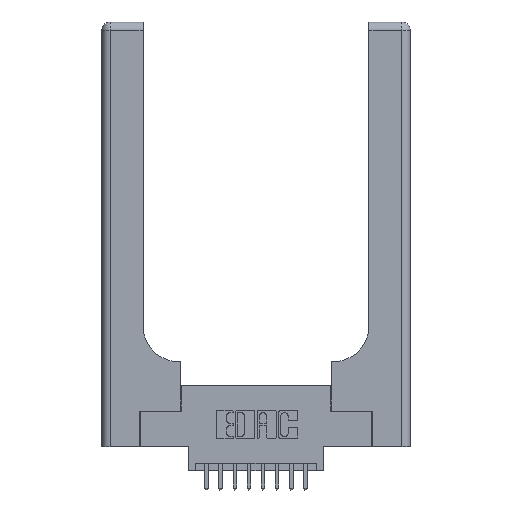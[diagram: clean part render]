
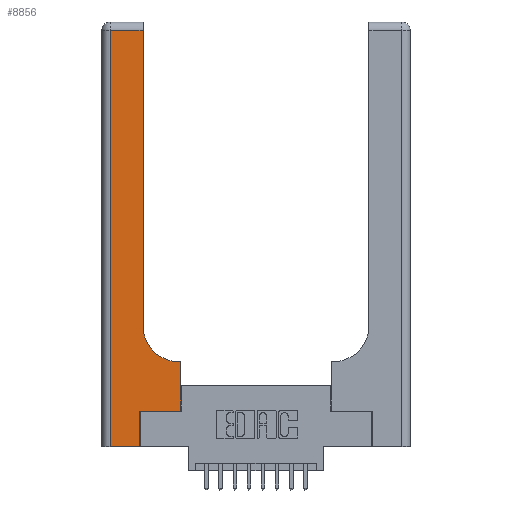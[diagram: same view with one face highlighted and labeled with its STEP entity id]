
A CAD part, top view. The second image highlights one B-rep face of the part: STEP entity #8856.
In plain terms, the highlighted planar face has unit normal (0, 0, 1).
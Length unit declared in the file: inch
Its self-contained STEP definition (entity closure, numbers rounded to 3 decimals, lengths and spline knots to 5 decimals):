
#117 = DIRECTION ( 'NONE',  ( 0., -1., 0. ) ) ;
#145 = CARTESIAN_POINT ( 'NONE',  ( 0.2915, 3., 0.37 ) ) ;
#798 = DIRECTION ( 'NONE',  ( -1., 0., 0. ) ) ;
#891 = VERTEX_POINT ( 'NONE', #4450 ) ;
#1082 = ORIENTED_EDGE ( 'NONE', *, *, #5301, .T. ) ;
#1162 = PLANE ( 'NONE',  #9808 ) ;
#1988 = LINE ( 'NONE', #13821, #11573 ) ;
#2045 = VECTOR ( 'NONE', #13117, 39.37008 ) ;
#2128 = DIRECTION ( 'NONE',  ( 1., 0., 0. ) ) ;
#2146 = DIRECTION ( 'NONE',  ( 0., 0., -1. ) ) ;
#2162 = CARTESIAN_POINT ( 'NONE',  ( 0.5415, 0.85, 0.37 ) ) ;
#2391 = VERTEX_POINT ( 'NONE', #8652 ) ;
#2441 = ORIENTED_EDGE ( 'NONE', *, *, #9948, .T. ) ;
#2488 = VECTOR ( 'NONE', #12244, 39.37008 ) ;
#2704 = DIRECTION ( 'NONE',  ( 0., 1., 0. ) ) ;
#2963 = CARTESIAN_POINT ( 'NONE',  ( 0.06, 2.94, 0.37 ) ) ;
#2995 = ORIENTED_EDGE ( 'NONE', *, *, #10984, .T. ) ;
#3245 = EDGE_CURVE ( 'NONE', #11311, #9466, #4702, .T. ) ;
#4249 = CARTESIAN_POINT ( 'NONE',  ( 0.06, 0., 0.37 ) ) ;
#4450 = CARTESIAN_POINT ( 'NONE',  ( 0.269, 0.25, 0.37 ) ) ;
#4457 = CARTESIAN_POINT ( 'NONE',  ( 0., 2.94, 0.37 ) ) ;
#4702 = CIRCLE ( 'NONE', #12982, 0.25 ) ;
#4974 = DIRECTION ( 'NONE',  ( -1., 0., 0. ) ) ;
#5070 = CARTESIAN_POINT ( 'NONE',  ( 0.2915, 0.85, 0.37 ) ) ;
#5249 = CARTESIAN_POINT ( 'NONE',  ( 0.269, 0., 0.37 ) ) ;
#5293 = CARTESIAN_POINT ( 'NONE',  ( 0.5585, 0.25, 0.37 ) ) ;
#5301 = EDGE_CURVE ( 'NONE', #7174, #891, #6236, .T. ) ;
#5472 = ORIENTED_EDGE ( 'NONE', *, *, #3245, .T. ) ;
#5630 = DIRECTION ( 'NONE',  ( 0., 1., 0. ) ) ;
#5690 = CARTESIAN_POINT ( 'NONE',  ( 0., 0., 0.37 ) ) ;
#5772 = LINE ( 'NONE', #145, #11979 ) ;
#5844 = DIRECTION ( 'NONE',  ( 1., 0., 0. ) ) ;
#5846 = CARTESIAN_POINT ( 'NONE',  ( 0.2915, 0.6, 0.37 ) ) ;
#5911 = EDGE_CURVE ( 'NONE', #2391, #11311, #10860, .T. ) ;
#6059 = VERTEX_POINT ( 'NONE', #5293 ) ;
#6215 = VECTOR ( 'NONE', #14359, 39.37008 ) ;
#6236 = LINE ( 'NONE', #8531, #2488 ) ;
#6268 = EDGE_CURVE ( 'NONE', #7899, #6760, #14922, .T. ) ;
#6528 = ORIENTED_EDGE ( 'NONE', *, *, #5911, .T. ) ;
#6760 = VERTEX_POINT ( 'NONE', #2963 ) ;
#7079 = FACE_OUTER_BOUND ( 'NONE', #8393, .T. ) ;
#7174 = VERTEX_POINT ( 'NONE', #5249 ) ;
#7430 = CARTESIAN_POINT ( 'NONE',  ( 0., 3., 0.37 ) ) ;
#7899 = VERTEX_POINT ( 'NONE', #15357 ) ;
#8338 = CARTESIAN_POINT ( 'NONE',  ( 0.5415, 0.6, 0.37 ) ) ;
#8393 = EDGE_LOOP ( 'NONE', ( #2995, #11594, #15044, #2441, #1082, #15892, #14537, #6528, #5472 ) ) ;
#8531 = CARTESIAN_POINT ( 'NONE',  ( 0.269, 0., 0.37 ) ) ;
#8652 = CARTESIAN_POINT ( 'NONE',  ( 0.5585, 0.6, 0.37 ) ) ;
#8856 = ADVANCED_FACE ( 'NONE', ( #7079 ), #1162, .F. ) ;
#8884 = LINE ( 'NONE', #13044, #11981 ) ;
#9294 = VECTOR ( 'NONE', #5844, 39.37008 ) ;
#9466 = VERTEX_POINT ( 'NONE', #5070 ) ;
#9583 = CARTESIAN_POINT ( 'NONE',  ( 0.269, 0.25, 0.37 ) ) ;
#9808 = AXIS2_PLACEMENT_3D ( 'NONE', #7430, #12406, #4974 ) ;
#9948 = EDGE_CURVE ( 'NONE', #15198, #7174, #15312, .T. ) ;
#10682 = EDGE_CURVE ( 'NONE', #891, #6059, #12581, .T. ) ;
#10860 = LINE ( 'NONE', #5846, #13763 ) ;
#10984 = EDGE_CURVE ( 'NONE', #9466, #7899, #5772, .T. ) ;
#11311 = VERTEX_POINT ( 'NONE', #8338 ) ;
#11573 = VECTOR ( 'NONE', #117, 39.37008 ) ;
#11594 = ORIENTED_EDGE ( 'NONE', *, *, #6268, .T. ) ;
#11754 = EDGE_CURVE ( 'NONE', #6059, #2391, #8884, .T. ) ;
#11979 = VECTOR ( 'NONE', #2704, 39.37008 ) ;
#11981 = VECTOR ( 'NONE', #5630, 39.37008 ) ;
#12244 = DIRECTION ( 'NONE',  ( 0., 1., 0. ) ) ;
#12406 = DIRECTION ( 'NONE',  ( 0., 0., -1. ) ) ;
#12581 = LINE ( 'NONE', #9583, #9294 ) ;
#12796 = EDGE_CURVE ( 'NONE', #6760, #15198, #1988, .T. ) ;
#12982 = AXIS2_PLACEMENT_3D ( 'NONE', #2162, #2146, #2128 ) ;
#13044 = CARTESIAN_POINT ( 'NONE',  ( 0.5585, 0.25, 0.37 ) ) ;
#13117 = DIRECTION ( 'NONE',  ( -1., 0., 0. ) ) ;
#13763 = VECTOR ( 'NONE', #798, 39.37008 ) ;
#13821 = CARTESIAN_POINT ( 'NONE',  ( 0.06, 3., 0.37 ) ) ;
#14359 = DIRECTION ( 'NONE',  ( 1., 0., 0. ) ) ;
#14537 = ORIENTED_EDGE ( 'NONE', *, *, #11754, .T. ) ;
#14922 = LINE ( 'NONE', #4457, #2045 ) ;
#15044 = ORIENTED_EDGE ( 'NONE', *, *, #12796, .T. ) ;
#15198 = VERTEX_POINT ( 'NONE', #4249 ) ;
#15312 = LINE ( 'NONE', #5690, #6215 ) ;
#15357 = CARTESIAN_POINT ( 'NONE',  ( 0.2915, 2.94, 0.37 ) ) ;
#15892 = ORIENTED_EDGE ( 'NONE', *, *, #10682, .T. ) ;
